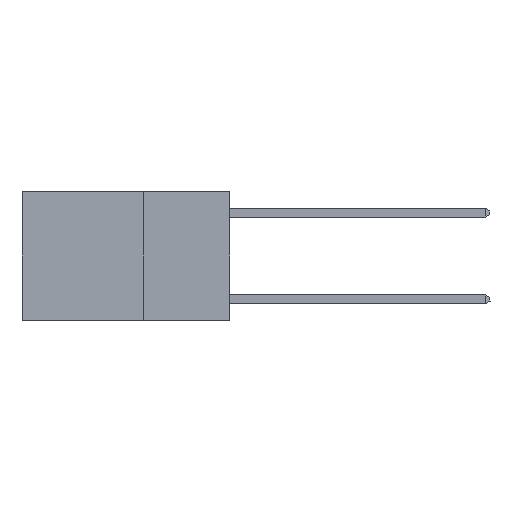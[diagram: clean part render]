
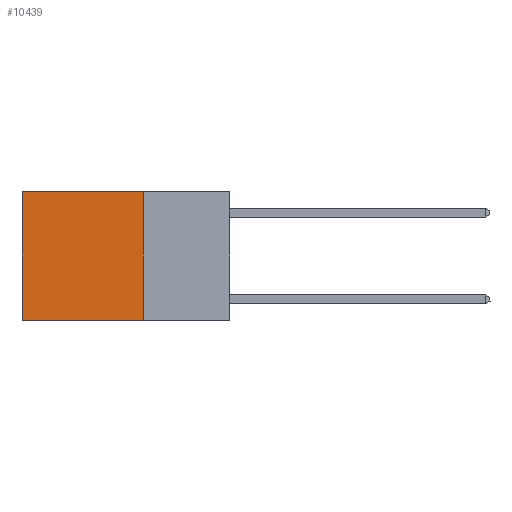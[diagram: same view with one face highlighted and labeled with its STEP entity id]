
A CAD part, left-side view. The second image highlights one B-rep face of the part: STEP entity #10439.
In plain terms, the highlighted planar face has unit normal (-1, 0, 0).
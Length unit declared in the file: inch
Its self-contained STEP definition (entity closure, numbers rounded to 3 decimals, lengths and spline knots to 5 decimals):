
#353 = VERTEX_POINT ( 'NONE', #671 ) ;
#671 = CARTESIAN_POINT ( 'NONE',  ( 0.2625, 0.6, -0.37 ) ) ;
#1215 = CARTESIAN_POINT ( 'NONE',  ( 0.2625, 0.25, 0. ) ) ;
#1433 = LINE ( 'NONE', #1607, #7928 ) ;
#1607 = CARTESIAN_POINT ( 'NONE',  ( 0.2625, 0.25, 0. ) ) ;
#1676 = CARTESIAN_POINT ( 'NONE',  ( 0.2625, 0.25, 0. ) ) ;
#1966 = DIRECTION ( 'NONE',  ( 0., 0., -1. ) ) ;
#1995 = EDGE_CURVE ( 'NONE', #15940, #353, #5848, .T. ) ;
#2108 = FACE_OUTER_BOUND ( 'NONE', #14283, .T. ) ;
#2246 = ORIENTED_EDGE ( 'NONE', *, *, #1995, .F. ) ;
#2512 = VECTOR ( 'NONE', #7973, 39.37008 ) ;
#2603 = ORIENTED_EDGE ( 'NONE', *, *, #12150, .T. ) ;
#3132 = DIRECTION ( 'NONE',  ( 1., 0., 0. ) ) ;
#3288 = VERTEX_POINT ( 'NONE', #1215 ) ;
#4193 = CARTESIAN_POINT ( 'NONE',  ( 0.2625, 0.25, -0.37 ) ) ;
#4421 = EDGE_CURVE ( 'NONE', #8971, #353, #10827, .T. ) ;
#5154 = CARTESIAN_POINT ( 'NONE',  ( 0.2625, 0.6, 0. ) ) ;
#5413 = VECTOR ( 'NONE', #6834, 39.37008 ) ;
#5848 = LINE ( 'NONE', #4193, #11482 ) ;
#6834 = DIRECTION ( 'NONE',  ( 0., 0., -1. ) ) ;
#7125 = ORIENTED_EDGE ( 'NONE', *, *, #14411, .F. ) ;
#7928 = VECTOR ( 'NONE', #13199, 39.37008 ) ;
#7973 = DIRECTION ( 'NONE',  ( 0., 0., -1. ) ) ;
#8889 = AXIS2_PLACEMENT_3D ( 'NONE', #13552, #3132, #1966 ) ;
#8971 = VERTEX_POINT ( 'NONE', #5154 ) ;
#10233 = ORIENTED_EDGE ( 'NONE', *, *, #4421, .T. ) ;
#10439 = ADVANCED_FACE ( 'NONE', ( #2108 ), #14975, .F. ) ;
#10827 = LINE ( 'NONE', #16638, #2512 ) ;
#11482 = VECTOR ( 'NONE', #14563, 39.37008 ) ;
#12150 = EDGE_CURVE ( 'NONE', #3288, #8971, #1433, .T. ) ;
#12303 = LINE ( 'NONE', #1676, #5413 ) ;
#13199 = DIRECTION ( 'NONE',  ( 0., 1., 0. ) ) ;
#13552 = CARTESIAN_POINT ( 'NONE',  ( 0.2625, 0.25, 0. ) ) ;
#14283 = EDGE_LOOP ( 'NONE', ( #10233, #2246, #7125, #2603 ) ) ;
#14411 = EDGE_CURVE ( 'NONE', #3288, #15940, #12303, .T. ) ;
#14563 = DIRECTION ( 'NONE',  ( 0., 1., 0. ) ) ;
#14630 = CARTESIAN_POINT ( 'NONE',  ( 0.2625, 0.25, -0.37 ) ) ;
#14975 = PLANE ( 'NONE',  #8889 ) ;
#15940 = VERTEX_POINT ( 'NONE', #14630 ) ;
#16638 = CARTESIAN_POINT ( 'NONE',  ( 0.2625, 0.6, 0. ) ) ;
